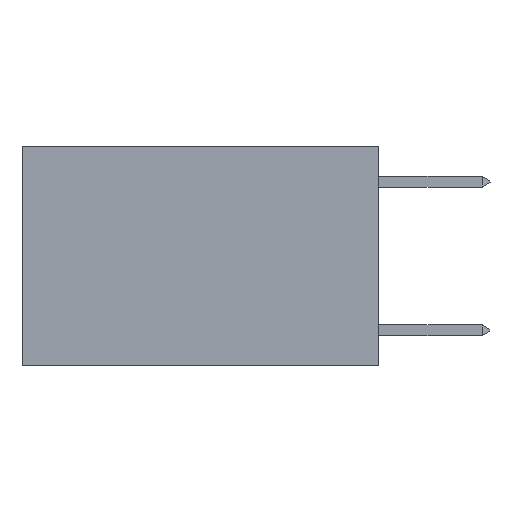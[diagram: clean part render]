
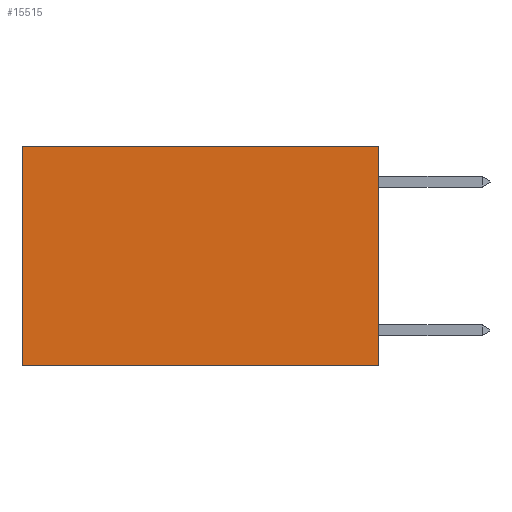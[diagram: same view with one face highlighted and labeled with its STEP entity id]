
A CAD part, left-side view. The second image highlights one B-rep face of the part: STEP entity #15515.
In plain terms, the highlighted planar face has unit normal (-1, 0, 0).
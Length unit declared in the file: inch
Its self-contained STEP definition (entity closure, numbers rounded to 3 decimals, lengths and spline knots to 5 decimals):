
#1036 = VECTOR ( 'NONE', #5177, 39.37008 ) ;
#1482 = EDGE_CURVE ( 'NONE', #18564, #20720, #8618, .T. ) ;
#2911 = FACE_OUTER_BOUND ( 'NONE', #13722, .T. ) ;
#3182 = ORIENTED_EDGE ( 'NONE', *, *, #22456, .T. ) ;
#4501 = DIRECTION ( 'NONE',  ( 0., 0., -1. ) ) ;
#4591 = ORIENTED_EDGE ( 'NONE', *, *, #14839, .T. ) ;
#5177 = DIRECTION ( 'NONE',  ( 0., 1., 0. ) ) ;
#5875 = CARTESIAN_POINT ( 'NONE',  ( 0.2625, 0., -0.37 ) ) ;
#6534 = VECTOR ( 'NONE', #7168, 39.37008 ) ;
#7168 = DIRECTION ( 'NONE',  ( 0., 0., -1. ) ) ;
#8573 = DIRECTION ( 'NONE',  ( 0., 0., -1. ) ) ;
#8618 = LINE ( 'NONE', #14138, #1036 ) ;
#9019 = LINE ( 'NONE', #23939, #6534 ) ;
#10280 = CARTESIAN_POINT ( 'NONE',  ( 0.2625, 0.6, 0. ) ) ;
#10601 = VECTOR ( 'NONE', #22552, 39.37008 ) ;
#12186 = VERTEX_POINT ( 'NONE', #19014 ) ;
#13130 = CARTESIAN_POINT ( 'NONE',  ( 0.2625, 0., 0. ) ) ;
#13722 = EDGE_LOOP ( 'NONE', ( #3182, #22098, #16546, #4591 ) ) ;
#14138 = CARTESIAN_POINT ( 'NONE',  ( 0.2625, 0., -0.37 ) ) ;
#14628 = CARTESIAN_POINT ( 'NONE',  ( 0.2625, 0.6, -0.37 ) ) ;
#14839 = EDGE_CURVE ( 'NONE', #21485, #12186, #22311, .T. ) ;
#15515 = ADVANCED_FACE ( 'NONE', ( #2911 ), #15997, .F. ) ;
#15997 = PLANE ( 'NONE',  #17797 ) ;
#16111 = DIRECTION ( 'NONE',  ( 1., 0., 0. ) ) ;
#16546 = ORIENTED_EDGE ( 'NONE', *, *, #20663, .F. ) ;
#16560 = CARTESIAN_POINT ( 'NONE',  ( 0.2625, 0., 0. ) ) ;
#17797 = AXIS2_PLACEMENT_3D ( 'NONE', #21265, #16111, #4501 ) ;
#18564 = VERTEX_POINT ( 'NONE', #5875 ) ;
#19014 = CARTESIAN_POINT ( 'NONE',  ( 0.2625, 0.6, 0. ) ) ;
#20056 = LINE ( 'NONE', #10280, #23872 ) ;
#20663 = EDGE_CURVE ( 'NONE', #21485, #18564, #9019, .T. ) ;
#20720 = VERTEX_POINT ( 'NONE', #14628 ) ;
#21265 = CARTESIAN_POINT ( 'NONE',  ( 0.2625, 0., 0. ) ) ;
#21485 = VERTEX_POINT ( 'NONE', #16560 ) ;
#22098 = ORIENTED_EDGE ( 'NONE', *, *, #1482, .F. ) ;
#22311 = LINE ( 'NONE', #13130, #10601 ) ;
#22456 = EDGE_CURVE ( 'NONE', #12186, #20720, #20056, .T. ) ;
#22552 = DIRECTION ( 'NONE',  ( 0., 1., 0. ) ) ;
#23872 = VECTOR ( 'NONE', #8573, 39.37008 ) ;
#23939 = CARTESIAN_POINT ( 'NONE',  ( 0.2625, 0., 0. ) ) ;
